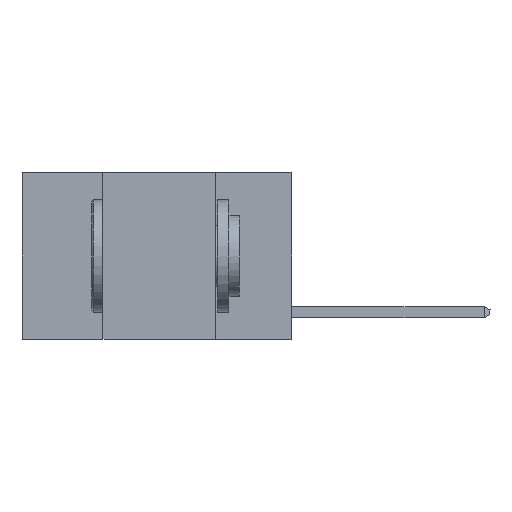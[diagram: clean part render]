
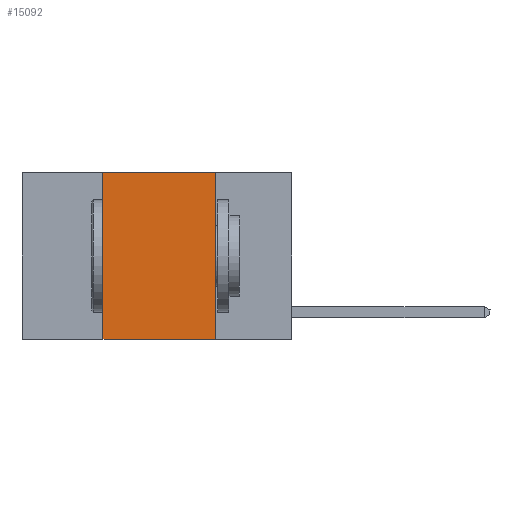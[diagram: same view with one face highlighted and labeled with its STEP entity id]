
A CAD part, left-side view. The second image highlights one B-rep face of the part: STEP entity #15092.
In plain terms, the highlighted planar face has unit normal (-1, 0, 0).
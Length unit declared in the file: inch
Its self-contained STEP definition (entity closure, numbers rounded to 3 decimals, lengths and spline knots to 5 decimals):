
#1018 = EDGE_LOOP ( 'NONE', ( #16790, #2641, #26767, #17186 ) ) ;
#2641 = ORIENTED_EDGE ( 'NONE', *, *, #21172, .F. ) ;
#4191 = AXIS2_PLACEMENT_3D ( 'NONE', #17210, #12767, #8743 ) ;
#4622 = LINE ( 'NONE', #15139, #18273 ) ;
#6025 = CARTESIAN_POINT ( 'NONE',  ( 0., 0.42, 0. ) ) ;
#8743 = DIRECTION ( 'NONE',  ( 0., 0., -1. ) ) ;
#9911 = VECTOR ( 'NONE', #14732, 39.37008 ) ;
#11246 = CARTESIAN_POINT ( 'NONE',  ( 0., 0.42, 0. ) ) ;
#11569 = LINE ( 'NONE', #6025, #27401 ) ;
#11783 = CARTESIAN_POINT ( 'NONE',  ( 0., 0.17, 0. ) ) ;
#12409 = CARTESIAN_POINT ( 'NONE',  ( 0., 0.6, -0.37 ) ) ;
#12767 = DIRECTION ( 'NONE',  ( 1., 0., 0. ) ) ;
#13622 = VERTEX_POINT ( 'NONE', #11246 ) ;
#14732 = DIRECTION ( 'NONE',  ( 0., -1., 0. ) ) ;
#15092 = ADVANCED_FACE ( 'NONE', ( #20500 ), #21884, .F. ) ;
#15139 = CARTESIAN_POINT ( 'NONE',  ( 0., 0.17, 0. ) ) ;
#16364 = DIRECTION ( 'NONE',  ( 0., 0., -1. ) ) ;
#16790 = ORIENTED_EDGE ( 'NONE', *, *, #18127, .F. ) ;
#17186 = ORIENTED_EDGE ( 'NONE', *, *, #23616, .T. ) ;
#17210 = CARTESIAN_POINT ( 'NONE',  ( 0., 0.6, 0. ) ) ;
#18127 = EDGE_CURVE ( 'NONE', #19432, #27995, #4622, .T. ) ;
#18144 = CARTESIAN_POINT ( 'NONE',  ( 0., 0.42, -0.37 ) ) ;
#18273 = VECTOR ( 'NONE', #16364, 39.37008 ) ;
#19432 = VERTEX_POINT ( 'NONE', #11783 ) ;
#19883 = LINE ( 'NONE', #21174, #9911 ) ;
#20500 = FACE_OUTER_BOUND ( 'NONE', #1018, .T. ) ;
#21060 = LINE ( 'NONE', #12409, #22438 ) ;
#21172 = EDGE_CURVE ( 'NONE', #13622, #19432, #19883, .T. ) ;
#21174 = CARTESIAN_POINT ( 'NONE',  ( 0., 0.6, 0. ) ) ;
#21884 = PLANE ( 'NONE',  #4191 ) ;
#22438 = VECTOR ( 'NONE', #26163, 39.37008 ) ;
#23303 = CARTESIAN_POINT ( 'NONE',  ( 0., 0.17, -0.37 ) ) ;
#23616 = EDGE_CURVE ( 'NONE', #26144, #27995, #21060, .T. ) ;
#26144 = VERTEX_POINT ( 'NONE', #18144 ) ;
#26163 = DIRECTION ( 'NONE',  ( 0., -1., 0. ) ) ;
#26355 = EDGE_CURVE ( 'NONE', #26144, #13622, #11569, .T. ) ;
#26508 = DIRECTION ( 'NONE',  ( 0., 0., 1. ) ) ;
#26767 = ORIENTED_EDGE ( 'NONE', *, *, #26355, .F. ) ;
#27401 = VECTOR ( 'NONE', #26508, 39.37008 ) ;
#27995 = VERTEX_POINT ( 'NONE', #23303 ) ;
